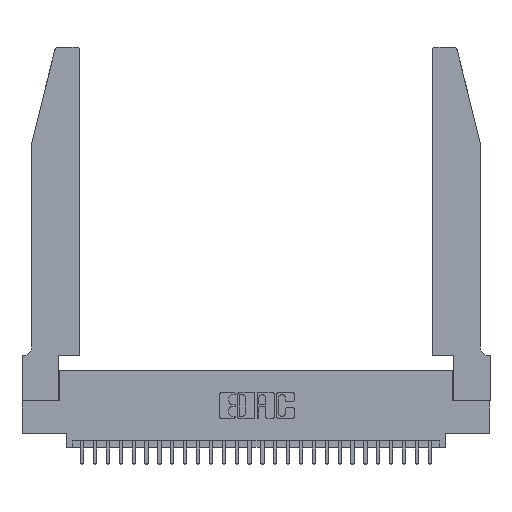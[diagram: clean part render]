
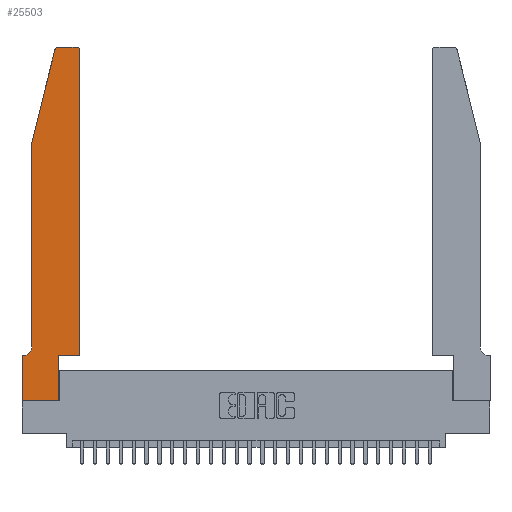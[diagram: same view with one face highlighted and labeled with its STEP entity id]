
A CAD part, top view. The second image highlights one B-rep face of the part: STEP entity #25503.
In plain terms, the highlighted planar face has unit normal (0, 0, 1).
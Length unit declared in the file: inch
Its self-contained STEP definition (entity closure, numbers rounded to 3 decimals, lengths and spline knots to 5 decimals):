
#179 = DIRECTION ( 'NONE',  ( 0., 0., 1. ) ) ;
#307 = ORIENTED_EDGE ( 'NONE', *, *, #1085, .T. ) ;
#351 = VECTOR ( 'NONE', #913, 39.37008 ) ;
#420 = CARTESIAN_POINT ( 'NONE',  ( 0.0755, 2., 0.37 ) ) ;
#913 = DIRECTION ( 'NONE',  ( 1., 0., 0. ) ) ;
#988 = CARTESIAN_POINT ( 'NONE',  ( 0.0755, 0.42, 0.37 ) ) ;
#1085 = EDGE_CURVE ( 'NONE', #21641, #28249, #28609, .T. ) ;
#1399 = CARTESIAN_POINT ( 'NONE',  ( 0.4505, 0.35, 0.37 ) ) ;
#1499 = DIRECTION ( 'NONE',  ( 0., 0., 1. ) ) ;
#2872 = LINE ( 'NONE', #22788, #14960 ) ;
#3451 = CARTESIAN_POINT ( 'NONE',  ( 0.4505, 0.35, 0.37 ) ) ;
#4451 = AXIS2_PLACEMENT_3D ( 'NONE', #15100, #1499, #17313 ) ;
#4462 = EDGE_CURVE ( 'NONE', #23592, #27883, #6385, .T. ) ;
#4728 = CARTESIAN_POINT ( 'NONE',  ( 0.2605, 2.75, 0.37 ) ) ;
#5180 = EDGE_CURVE ( 'NONE', #6651, #26564, #21394, .T. ) ;
#6093 = CIRCLE ( 'NONE', #11784, 0.07 ) ;
#6385 = CIRCLE ( 'NONE', #9065, 0.03 ) ;
#6587 = VECTOR ( 'NONE', #22095, 39.37008 ) ;
#6651 = VERTEX_POINT ( 'NONE', #7690 ) ;
#7314 = DIRECTION ( 'NONE',  ( 0., -1., 0. ) ) ;
#7690 = CARTESIAN_POINT ( 'NONE',  ( 0.2865, 0., 0.37 ) ) ;
#7772 = CARTESIAN_POINT ( 'NONE',  ( 0.284, 2.75, 0.37 ) ) ;
#8015 = EDGE_CURVE ( 'NONE', #15283, #25349, #12028, .T. ) ;
#8208 = ORIENTED_EDGE ( 'NONE', *, *, #26884, .T. ) ;
#9065 = AXIS2_PLACEMENT_3D ( 'NONE', #26469, #13441, #28640 ) ;
#9287 = CARTESIAN_POINT ( 'NONE',  ( 0., 0.35, 0.37 ) ) ;
#9694 = CIRCLE ( 'NONE', #13033, 0.03 ) ;
#10255 = ORIENTED_EDGE ( 'NONE', *, *, #11346, .T. ) ;
#10368 = VECTOR ( 'NONE', #22286, 39.37008 ) ;
#10924 = DIRECTION ( 'NONE',  ( 0., 0., -1. ) ) ;
#11346 = EDGE_CURVE ( 'NONE', #21805, #11677, #9694, .T. ) ;
#11388 = CARTESIAN_POINT ( 'NONE',  ( 0.0055, 0.35, 0.37 ) ) ;
#11527 = DIRECTION ( 'NONE',  ( -1., 0., 0. ) ) ;
#11677 = VERTEX_POINT ( 'NONE', #28059 ) ;
#11784 = AXIS2_PLACEMENT_3D ( 'NONE', #24015, #10924, #26203 ) ;
#12028 = LINE ( 'NONE', #420, #16521 ) ;
#12876 = CARTESIAN_POINT ( 'NONE',  ( 0.0755, 2., 0.37 ) ) ;
#13033 = AXIS2_PLACEMENT_3D ( 'NONE', #13836, #179, #16064 ) ;
#13392 = EDGE_CURVE ( 'NONE', #28249, #17057, #2872, .T. ) ;
#13441 = DIRECTION ( 'NONE',  ( 0., 0., 1. ) ) ;
#13449 = CARTESIAN_POINT ( 'NONE',  ( 0.0755, 2., 0.37 ) ) ;
#13836 = CARTESIAN_POINT ( 'NONE',  ( 0.4205, 2.72, 0.37 ) ) ;
#13986 = LINE ( 'NONE', #4728, #19806 ) ;
#14060 = DIRECTION ( 'NONE',  ( 0., -1., 0. ) ) ;
#14255 = CARTESIAN_POINT ( 'NONE',  ( 0.2865, 0.35, 0.37 ) ) ;
#14396 = CARTESIAN_POINT ( 'NONE',  ( 0.4505, 2.72, 0.37 ) ) ;
#14909 = CARTESIAN_POINT ( 'NONE',  ( 0., 0., 0.37 ) ) ;
#14960 = VECTOR ( 'NONE', #7314, 39.37008 ) ;
#15100 = CARTESIAN_POINT ( 'NONE',  ( 0., 0.35, 0.37 ) ) ;
#15137 = ORIENTED_EDGE ( 'NONE', *, *, #19310, .T. ) ;
#15283 = VERTEX_POINT ( 'NONE', #13449 ) ;
#15626 = EDGE_LOOP ( 'NONE', ( #15137, #22946, #26059, #21541, #8208, #307, #16644, #24411, #17026, #20558, #18221, #10255 ) ) ;
#16064 = DIRECTION ( 'NONE',  ( 1., 0., 0. ) ) ;
#16521 = VECTOR ( 'NONE', #14060, 39.37008 ) ;
#16644 = ORIENTED_EDGE ( 'NONE', *, *, #13392, .T. ) ;
#17026 = ORIENTED_EDGE ( 'NONE', *, *, #5180, .T. ) ;
#17057 = VERTEX_POINT ( 'NONE', #19342 ) ;
#17313 = DIRECTION ( 'NONE',  ( 1., 0., 0. ) ) ;
#17934 = CARTESIAN_POINT ( 'NONE',  ( 0.0755, 0.35, 0.37 ) ) ;
#18221 = ORIENTED_EDGE ( 'NONE', *, *, #21930, .T. ) ;
#19292 = DIRECTION ( 'NONE',  ( 1., 0., 0. ) ) ;
#19310 = EDGE_CURVE ( 'NONE', #11677, #23592, #13986, .T. ) ;
#19342 = CARTESIAN_POINT ( 'NONE',  ( 0., 0., 0.37 ) ) ;
#19806 = VECTOR ( 'NONE', #11527, 39.37008 ) ;
#20099 = CARTESIAN_POINT ( 'NONE',  ( 0.2865, 0.35, 0.37 ) ) ;
#20558 = ORIENTED_EDGE ( 'NONE', *, *, #26630, .T. ) ;
#21339 = VECTOR ( 'NONE', #19292, 39.37008 ) ;
#21357 = DIRECTION ( 'NONE',  ( 0., 1., 0. ) ) ;
#21394 = LINE ( 'NONE', #20099, #10368 ) ;
#21541 = ORIENTED_EDGE ( 'NONE', *, *, #8015, .T. ) ;
#21641 = VERTEX_POINT ( 'NONE', #11388 ) ;
#21805 = VERTEX_POINT ( 'NONE', #14396 ) ;
#21819 = FACE_OUTER_BOUND ( 'NONE', #15626, .T. ) ;
#21930 = EDGE_CURVE ( 'NONE', #27365, #21805, #22756, .T. ) ;
#22095 = DIRECTION ( 'NONE',  ( -1., 0., 0. ) ) ;
#22286 = DIRECTION ( 'NONE',  ( 0., 1., 0. ) ) ;
#22756 = LINE ( 'NONE', #3451, #28488 ) ;
#22771 = LINE ( 'NONE', #23187, #351 ) ;
#22788 = CARTESIAN_POINT ( 'NONE',  ( 0., 0., 0.37 ) ) ;
#22946 = ORIENTED_EDGE ( 'NONE', *, *, #4462, .T. ) ;
#23162 = LINE ( 'NONE', #12876, #26871 ) ;
#23187 = CARTESIAN_POINT ( 'NONE',  ( 0.4505, 0.35, 0.37 ) ) ;
#23592 = VERTEX_POINT ( 'NONE', #7772 ) ;
#23712 = PLANE ( 'NONE',  #4451 ) ;
#24015 = CARTESIAN_POINT ( 'NONE',  ( 0.0055, 0.42, 0.37 ) ) ;
#24411 = ORIENTED_EDGE ( 'NONE', *, *, #28041, .T. ) ;
#25349 = VERTEX_POINT ( 'NONE', #988 ) ;
#25503 = ADVANCED_FACE ( 'NONE', ( #21819 ), #23712, .T. ) ;
#25512 = EDGE_CURVE ( 'NONE', #27883, #15283, #23162, .T. ) ;
#25984 = DIRECTION ( 'NONE',  ( -0.239, -0.971, 0. ) ) ;
#26059 = ORIENTED_EDGE ( 'NONE', *, *, #25512, .T. ) ;
#26203 = DIRECTION ( 'NONE',  ( -1., 0., 0. ) ) ;
#26469 = CARTESIAN_POINT ( 'NONE',  ( 0.284, 2.72, 0.37 ) ) ;
#26564 = VERTEX_POINT ( 'NONE', #14255 ) ;
#26630 = EDGE_CURVE ( 'NONE', #26564, #27365, #22771, .T. ) ;
#26871 = VECTOR ( 'NONE', #25984, 39.37008 ) ;
#26884 = EDGE_CURVE ( 'NONE', #25349, #21641, #6093, .T. ) ;
#27066 = LINE ( 'NONE', #14909, #21339 ) ;
#27365 = VERTEX_POINT ( 'NONE', #1399 ) ;
#27883 = VERTEX_POINT ( 'NONE', #28134 ) ;
#28041 = EDGE_CURVE ( 'NONE', #17057, #6651, #27066, .T. ) ;
#28059 = CARTESIAN_POINT ( 'NONE',  ( 0.4205, 2.75, 0.37 ) ) ;
#28134 = CARTESIAN_POINT ( 'NONE',  ( 0.25487, 2.72718, 0.37 ) ) ;
#28249 = VERTEX_POINT ( 'NONE', #9287 ) ;
#28488 = VECTOR ( 'NONE', #21357, 39.37008 ) ;
#28609 = LINE ( 'NONE', #17934, #6587 ) ;
#28640 = DIRECTION ( 'NONE',  ( 1., 0., 0. ) ) ;
